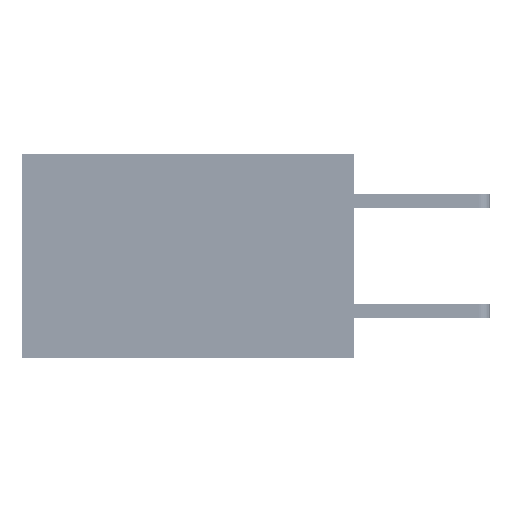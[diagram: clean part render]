
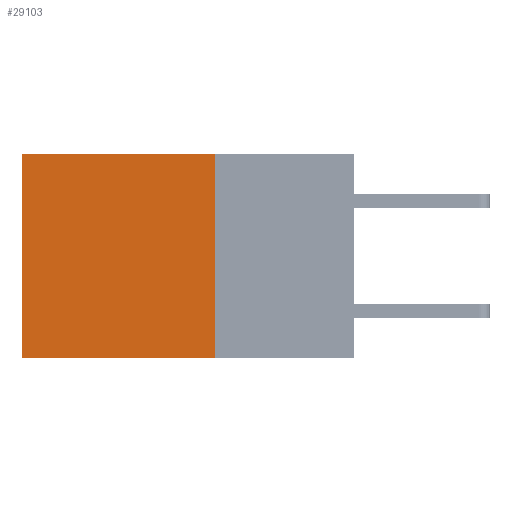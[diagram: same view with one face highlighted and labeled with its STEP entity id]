
A CAD part, left-side view. The second image highlights one B-rep face of the part: STEP entity #29103.
In plain terms, the highlighted planar face has unit normal (-1, 0, 0).
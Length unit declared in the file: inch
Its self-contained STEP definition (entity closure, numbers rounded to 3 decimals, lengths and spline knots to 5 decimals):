
#1094 = AXIS2_PLACEMENT_3D ( 'NONE', #9615, #22997, #2069 ) ;
#2069 = DIRECTION ( 'NONE',  ( 0., 0., -1. ) ) ;
#2936 = CARTESIAN_POINT ( 'NONE',  ( 0.2875, 0.6, 0. ) ) ;
#3118 = VECTOR ( 'NONE', #34622, 39.37008 ) ;
#4579 = LINE ( 'NONE', #39080, #26884 ) ;
#6441 = EDGE_LOOP ( 'NONE', ( #23819, #17654, #28916, #22280 ) ) ;
#7452 = LINE ( 'NONE', #24400, #3118 ) ;
#8340 = EDGE_CURVE ( 'NONE', #29160, #34226, #7452, .T. ) ;
#8574 = CARTESIAN_POINT ( 'NONE',  ( 0.2875, 0.25, -0.37 ) ) ;
#9348 = DIRECTION ( 'NONE',  ( 0., 1., 0. ) ) ;
#9615 = CARTESIAN_POINT ( 'NONE',  ( 0.2875, 0.25, 0. ) ) ;
#9789 = VERTEX_POINT ( 'NONE', #8574 ) ;
#12960 = PLANE ( 'NONE',  #1094 ) ;
#13627 = CARTESIAN_POINT ( 'NONE',  ( 0.2875, 0.25, 0. ) ) ;
#14938 = LINE ( 'NONE', #27626, #41681 ) ;
#17654 = ORIENTED_EDGE ( 'NONE', *, *, #35816, .F. ) ;
#22280 = ORIENTED_EDGE ( 'NONE', *, *, #33009, .T. ) ;
#22521 = CARTESIAN_POINT ( 'NONE',  ( 0.2875, 0.25, 0. ) ) ;
#22633 = EDGE_CURVE ( 'NONE', #37873, #9789, #14938, .T. ) ;
#22997 = DIRECTION ( 'NONE',  ( 1., 0., 0. ) ) ;
#23819 = ORIENTED_EDGE ( 'NONE', *, *, #8340, .T. ) ;
#24400 = CARTESIAN_POINT ( 'NONE',  ( 0.2875, 0.6, 0. ) ) ;
#26884 = VECTOR ( 'NONE', #28421, 39.37008 ) ;
#27626 = CARTESIAN_POINT ( 'NONE',  ( 0.2875, 0.25, 0. ) ) ;
#28421 = DIRECTION ( 'NONE',  ( 0., 1., 0. ) ) ;
#28916 = ORIENTED_EDGE ( 'NONE', *, *, #22633, .F. ) ;
#29103 = ADVANCED_FACE ( 'NONE', ( #33218 ), #12960, .F. ) ;
#29160 = VERTEX_POINT ( 'NONE', #2936 ) ;
#33009 = EDGE_CURVE ( 'NONE', #37873, #29160, #39861, .T. ) ;
#33218 = FACE_OUTER_BOUND ( 'NONE', #6441, .T. ) ;
#34226 = VERTEX_POINT ( 'NONE', #38335 ) ;
#34503 = DIRECTION ( 'NONE',  ( 0., 0., -1. ) ) ;
#34622 = DIRECTION ( 'NONE',  ( 0., 0., -1. ) ) ;
#35816 = EDGE_CURVE ( 'NONE', #9789, #34226, #4579, .T. ) ;
#37873 = VERTEX_POINT ( 'NONE', #13627 ) ;
#38335 = CARTESIAN_POINT ( 'NONE',  ( 0.2875, 0.6, -0.37 ) ) ;
#39080 = CARTESIAN_POINT ( 'NONE',  ( 0.2875, 0.25, -0.37 ) ) ;
#39861 = LINE ( 'NONE', #22521, #42452 ) ;
#41681 = VECTOR ( 'NONE', #34503, 39.37008 ) ;
#42452 = VECTOR ( 'NONE', #9348, 39.37008 ) ;
